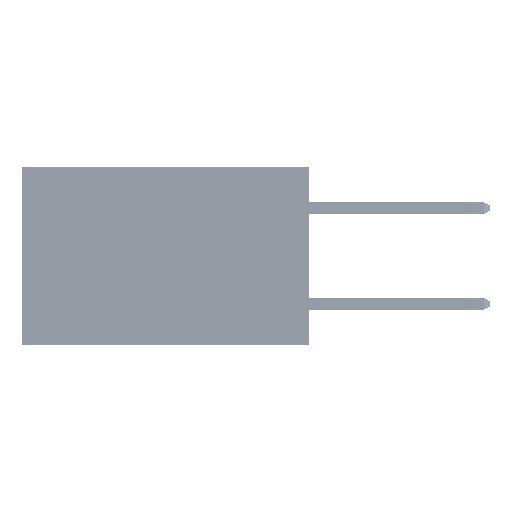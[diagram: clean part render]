
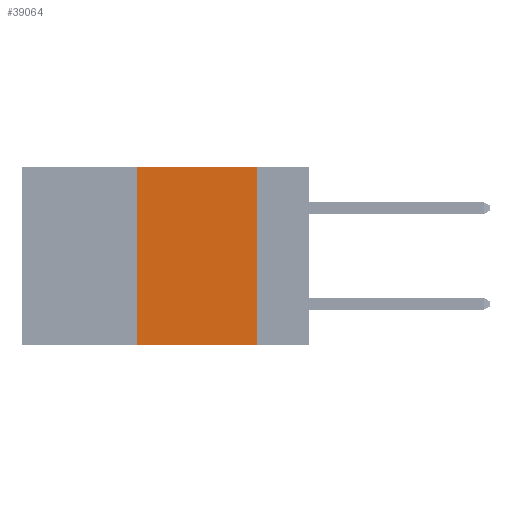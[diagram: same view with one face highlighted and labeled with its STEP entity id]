
A CAD part, left-side view. The second image highlights one B-rep face of the part: STEP entity #39064.
In plain terms, the highlighted planar face has unit normal (-1, 0, 0).
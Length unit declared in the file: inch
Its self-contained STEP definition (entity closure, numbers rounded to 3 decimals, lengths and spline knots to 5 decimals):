
#11 = CARTESIAN_POINT ( 'NONE',  ( 0., 0.11, 0. ) ) ;
#1953 = EDGE_LOOP ( 'NONE', ( #34613, #45882, #45245, #46178 ) ) ;
#2882 = EDGE_CURVE ( 'NONE', #26516, #40174, #23824, .T. ) ;
#2958 = VECTOR ( 'NONE', #29911, 39.37008 ) ;
#5560 = CARTESIAN_POINT ( 'NONE',  ( 0., 0.6, 0. ) ) ;
#9189 = DIRECTION ( 'NONE',  ( 1., 0., 0. ) ) ;
#9766 = VECTOR ( 'NONE', #16986, 39.37008 ) ;
#9884 = CARTESIAN_POINT ( 'NONE',  ( 0., 0.11, -0.37 ) ) ;
#13208 = DIRECTION ( 'NONE',  ( 0., 0., -1. ) ) ;
#13497 = EDGE_CURVE ( 'NONE', #37295, #30911, #25892, .T. ) ;
#13506 = DIRECTION ( 'NONE',  ( 0., 0., -1. ) ) ;
#16986 = DIRECTION ( 'NONE',  ( 0., 0., 1. ) ) ;
#17972 = FACE_OUTER_BOUND ( 'NONE', #1953, .T. ) ;
#21183 = DIRECTION ( 'NONE',  ( 0., -1., 0. ) ) ;
#21252 = VECTOR ( 'NONE', #21183, 39.37008 ) ;
#21345 = VECTOR ( 'NONE', #13506, 39.37008 ) ;
#23824 = LINE ( 'NONE', #11, #21345 ) ;
#25351 = EDGE_CURVE ( 'NONE', #30911, #26516, #29893, .T. ) ;
#25761 = CARTESIAN_POINT ( 'NONE',  ( 0., 0.6, -0.37 ) ) ;
#25892 = LINE ( 'NONE', #28757, #9766 ) ;
#26516 = VERTEX_POINT ( 'NONE', #37636 ) ;
#28757 = CARTESIAN_POINT ( 'NONE',  ( 0., 0.36, 0. ) ) ;
#29144 = PLANE ( 'NONE',  #36168 ) ;
#29893 = LINE ( 'NONE', #5560, #21252 ) ;
#29911 = DIRECTION ( 'NONE',  ( 0., -1., 0. ) ) ;
#30911 = VERTEX_POINT ( 'NONE', #34881 ) ;
#33000 = CARTESIAN_POINT ( 'NONE',  ( 0., 0.6, 0. ) ) ;
#34613 = ORIENTED_EDGE ( 'NONE', *, *, #2882, .F. ) ;
#34881 = CARTESIAN_POINT ( 'NONE',  ( 0., 0.36, 0. ) ) ;
#35386 = CARTESIAN_POINT ( 'NONE',  ( 0., 0.36, -0.37 ) ) ;
#36168 = AXIS2_PLACEMENT_3D ( 'NONE', #33000, #9189, #13208 ) ;
#36439 = LINE ( 'NONE', #25761, #2958 ) ;
#37295 = VERTEX_POINT ( 'NONE', #35386 ) ;
#37636 = CARTESIAN_POINT ( 'NONE',  ( 0., 0.11, 0. ) ) ;
#39064 = ADVANCED_FACE ( 'NONE', ( #17972 ), #29144, .F. ) ;
#40174 = VERTEX_POINT ( 'NONE', #9884 ) ;
#45245 = ORIENTED_EDGE ( 'NONE', *, *, #13497, .F. ) ;
#45882 = ORIENTED_EDGE ( 'NONE', *, *, #25351, .F. ) ;
#46178 = ORIENTED_EDGE ( 'NONE', *, *, #47789, .T. ) ;
#47789 = EDGE_CURVE ( 'NONE', #37295, #40174, #36439, .T. ) ;
